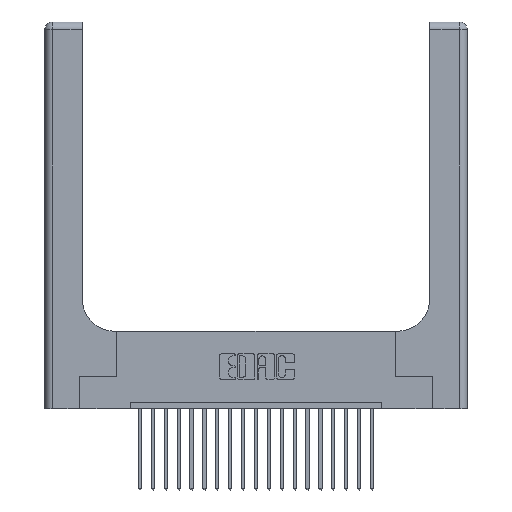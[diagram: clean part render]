
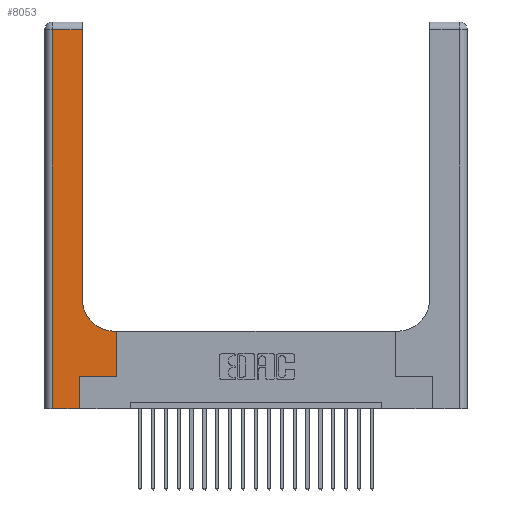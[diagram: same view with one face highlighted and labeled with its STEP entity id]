
A CAD part, top view. The second image highlights one B-rep face of the part: STEP entity #8053.
In plain terms, the highlighted planar face has unit normal (0, 0, 1).
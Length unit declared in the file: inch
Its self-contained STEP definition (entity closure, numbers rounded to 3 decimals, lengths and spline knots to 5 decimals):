
#1053 = CARTESIAN_POINT ( 'NONE',  ( 0.5585, 0.6, 0.37 ) ) ;
#1083 = CARTESIAN_POINT ( 'NONE',  ( 0.2915, 3., 0.37 ) ) ;
#1158 = VECTOR ( 'NONE', #7233, 39.37008 ) ;
#1537 = LINE ( 'NONE', #18783, #3926 ) ;
#1731 = DIRECTION ( 'NONE',  ( 0., 1., 0. ) ) ;
#1848 = LINE ( 'NONE', #4870, #16576 ) ;
#2193 = ORIENTED_EDGE ( 'NONE', *, *, #17319, .T. ) ;
#2541 = ORIENTED_EDGE ( 'NONE', *, *, #18216, .T. ) ;
#2552 = ORIENTED_EDGE ( 'NONE', *, *, #21438, .T. ) ;
#2741 = LINE ( 'NONE', #16194, #4580 ) ;
#2940 = VERTEX_POINT ( 'NONE', #18998 ) ;
#3077 = DIRECTION ( 'NONE',  ( 1., 0., 0. ) ) ;
#3727 = VECTOR ( 'NONE', #4643, 39.37008 ) ;
#3832 = CARTESIAN_POINT ( 'NONE',  ( 0., 2.94, 0.37 ) ) ;
#3926 = VECTOR ( 'NONE', #1731, 39.37008 ) ;
#4527 = ORIENTED_EDGE ( 'NONE', *, *, #4966, .T. ) ;
#4580 = VECTOR ( 'NONE', #11105, 39.37008 ) ;
#4643 = DIRECTION ( 'NONE',  ( 1., 0., 0. ) ) ;
#4781 = ORIENTED_EDGE ( 'NONE', *, *, #16679, .T. ) ;
#4870 = CARTESIAN_POINT ( 'NONE',  ( 0.06, 3., 0.37 ) ) ;
#4966 = EDGE_CURVE ( 'NONE', #18532, #2940, #20408, .T. ) ;
#5047 = VERTEX_POINT ( 'NONE', #7566 ) ;
#5174 = DIRECTION ( 'NONE',  ( 1., 0., 0. ) ) ;
#5248 = DIRECTION ( 'NONE',  ( 0., 0., -1. ) ) ;
#5750 = LINE ( 'NONE', #3832, #1158 ) ;
#5797 = FACE_OUTER_BOUND ( 'NONE', #16550, .T. ) ;
#6167 = AXIS2_PLACEMENT_3D ( 'NONE', #6632, #18720, #18945 ) ;
#6615 = EDGE_CURVE ( 'NONE', #5047, #18532, #1537, .T. ) ;
#6632 = CARTESIAN_POINT ( 'NONE',  ( 0., 3., 0.37 ) ) ;
#6757 = CARTESIAN_POINT ( 'NONE',  ( 0.269, 0.25, 0.37 ) ) ;
#7065 = LINE ( 'NONE', #11373, #18842 ) ;
#7233 = DIRECTION ( 'NONE',  ( -1., 0., 0. ) ) ;
#7566 = CARTESIAN_POINT ( 'NONE',  ( 0.269, 0., 0.37 ) ) ;
#8053 = ADVANCED_FACE ( 'NONE', ( #5797 ), #20649, .F. ) ;
#8247 = LINE ( 'NONE', #1083, #13463 ) ;
#8549 = LINE ( 'NONE', #11830, #17311 ) ;
#9808 = CARTESIAN_POINT ( 'NONE',  ( 0.269, 0.25, 0.37 ) ) ;
#9981 = EDGE_CURVE ( 'NONE', #17682, #16850, #1848, .T. ) ;
#10348 = CIRCLE ( 'NONE', #20803, 0.25 ) ;
#11105 = DIRECTION ( 'NONE',  ( -1., 0., 0. ) ) ;
#11373 = CARTESIAN_POINT ( 'NONE',  ( 0.5585, 0.25, 0.37 ) ) ;
#11662 = EDGE_CURVE ( 'NONE', #16033, #14633, #8247, .T. ) ;
#11830 = CARTESIAN_POINT ( 'NONE',  ( 0., 0., 0.37 ) ) ;
#12230 = ORIENTED_EDGE ( 'NONE', *, *, #11662, .T. ) ;
#13463 = VECTOR ( 'NONE', #21754, 39.37008 ) ;
#13727 = DIRECTION ( 'NONE',  ( 0., -1., 0. ) ) ;
#13830 = CARTESIAN_POINT ( 'NONE',  ( 0.2915, 2.94, 0.37 ) ) ;
#13883 = CARTESIAN_POINT ( 'NONE',  ( 0.5415, 0.85, 0.37 ) ) ;
#13975 = EDGE_CURVE ( 'NONE', #20554, #16033, #10348, .T. ) ;
#14633 = VERTEX_POINT ( 'NONE', #13830 ) ;
#15287 = ORIENTED_EDGE ( 'NONE', *, *, #6615, .T. ) ;
#15725 = CARTESIAN_POINT ( 'NONE',  ( 0.2915, 0.85, 0.37 ) ) ;
#16033 = VERTEX_POINT ( 'NONE', #15725 ) ;
#16194 = CARTESIAN_POINT ( 'NONE',  ( 0.2915, 0.6, 0.37 ) ) ;
#16509 = ORIENTED_EDGE ( 'NONE', *, *, #13975, .T. ) ;
#16550 = EDGE_LOOP ( 'NONE', ( #12230, #4781, #22510, #2552, #15287, #4527, #2193, #2541, #16509 ) ) ;
#16576 = VECTOR ( 'NONE', #13727, 39.37008 ) ;
#16679 = EDGE_CURVE ( 'NONE', #14633, #17682, #5750, .T. ) ;
#16850 = VERTEX_POINT ( 'NONE', #21863 ) ;
#17311 = VECTOR ( 'NONE', #3077, 39.37008 ) ;
#17319 = EDGE_CURVE ( 'NONE', #2940, #18478, #7065, .T. ) ;
#17682 = VERTEX_POINT ( 'NONE', #20983 ) ;
#18216 = EDGE_CURVE ( 'NONE', #18478, #20554, #2741, .T. ) ;
#18242 = DIRECTION ( 'NONE',  ( 0., 1., 0. ) ) ;
#18478 = VERTEX_POINT ( 'NONE', #1053 ) ;
#18532 = VERTEX_POINT ( 'NONE', #6757 ) ;
#18720 = DIRECTION ( 'NONE',  ( 0., 0., -1. ) ) ;
#18783 = CARTESIAN_POINT ( 'NONE',  ( 0.269, 0., 0.37 ) ) ;
#18842 = VECTOR ( 'NONE', #18242, 39.37008 ) ;
#18945 = DIRECTION ( 'NONE',  ( -1., 0., 0. ) ) ;
#18998 = CARTESIAN_POINT ( 'NONE',  ( 0.5585, 0.25, 0.37 ) ) ;
#20408 = LINE ( 'NONE', #9808, #3727 ) ;
#20554 = VERTEX_POINT ( 'NONE', #21424 ) ;
#20649 = PLANE ( 'NONE',  #6167 ) ;
#20803 = AXIS2_PLACEMENT_3D ( 'NONE', #13883, #5248, #5174 ) ;
#20983 = CARTESIAN_POINT ( 'NONE',  ( 0.06, 2.94, 0.37 ) ) ;
#21424 = CARTESIAN_POINT ( 'NONE',  ( 0.5415, 0.6, 0.37 ) ) ;
#21438 = EDGE_CURVE ( 'NONE', #16850, #5047, #8549, .T. ) ;
#21754 = DIRECTION ( 'NONE',  ( 0., 1., 0. ) ) ;
#21863 = CARTESIAN_POINT ( 'NONE',  ( 0.06, 0., 0.37 ) ) ;
#22510 = ORIENTED_EDGE ( 'NONE', *, *, #9981, .T. ) ;
